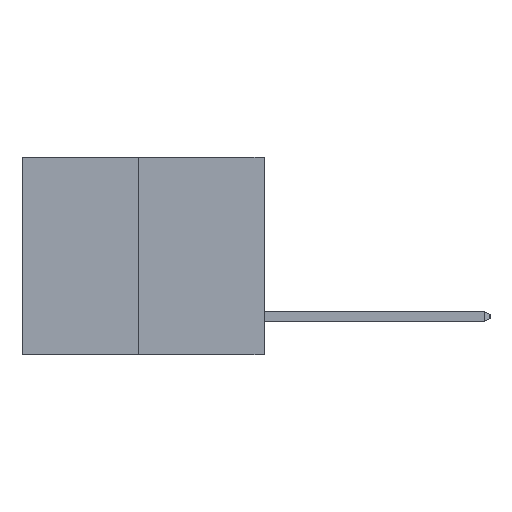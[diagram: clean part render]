
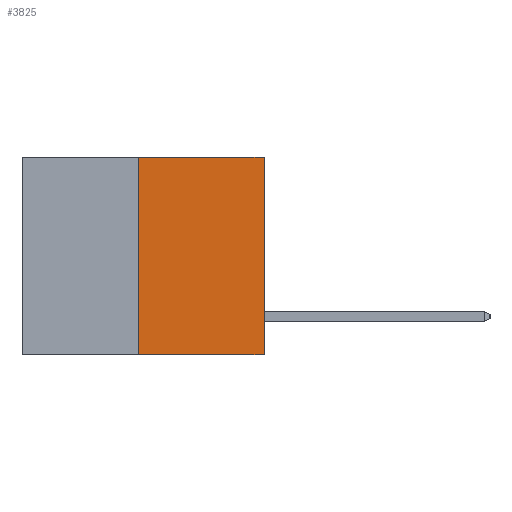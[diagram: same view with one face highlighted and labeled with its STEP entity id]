
A CAD part, left-side view. The second image highlights one B-rep face of the part: STEP entity #3825.
In plain terms, the highlighted planar face has unit normal (-1, 0, 0).
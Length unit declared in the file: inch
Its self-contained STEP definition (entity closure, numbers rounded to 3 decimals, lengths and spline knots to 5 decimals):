
#410 = ORIENTED_EDGE ( 'NONE', *, *, #24443, .F. ) ;
#1577 = CARTESIAN_POINT ( 'NONE',  ( 0., 0., 0. ) ) ;
#1878 = CARTESIAN_POINT ( 'NONE',  ( 0., 0.6, 0. ) ) ;
#3825 = ADVANCED_FACE ( 'NONE', ( #20770 ), #22673, .F. ) ;
#4087 = VECTOR ( 'NONE', #16035, 39.37008 ) ;
#5200 = VERTEX_POINT ( 'NONE', #17075 ) ;
#6329 = EDGE_LOOP ( 'NONE', ( #410, #20062, #16530, #17136 ) ) ;
#8845 = EDGE_CURVE ( 'NONE', #25019, #18686, #23222, .T. ) ;
#9444 = CARTESIAN_POINT ( 'NONE',  ( 0., 0.312, -0.49 ) ) ;
#9666 = CARTESIAN_POINT ( 'NONE',  ( 0., 0.6, -0.49 ) ) ;
#10748 = DIRECTION ( 'NONE',  ( 0., 0., 1. ) ) ;
#10788 = AXIS2_PLACEMENT_3D ( 'NONE', #15175, #15075, #24853 ) ;
#11562 = CARTESIAN_POINT ( 'NONE',  ( 0., 0.312, -0.49 ) ) ;
#12429 = VECTOR ( 'NONE', #10748, 39.37008 ) ;
#14781 = EDGE_CURVE ( 'NONE', #18686, #22151, #29075, .T. ) ;
#15075 = DIRECTION ( 'NONE',  ( 1., 0., 0. ) ) ;
#15175 = CARTESIAN_POINT ( 'NONE',  ( 0., 0.6, 0. ) ) ;
#15439 = LINE ( 'NONE', #1878, #19300 ) ;
#15719 = DIRECTION ( 'NONE',  ( 0., -1., 0. ) ) ;
#16035 = DIRECTION ( 'NONE',  ( 0., 0., 1. ) ) ;
#16257 = CARTESIAN_POINT ( 'NONE',  ( 0., 0., 0. ) ) ;
#16530 = ORIENTED_EDGE ( 'NONE', *, *, #14781, .T. ) ;
#17075 = CARTESIAN_POINT ( 'NONE',  ( 0., 0.312, 0. ) ) ;
#17136 = ORIENTED_EDGE ( 'NONE', *, *, #17328, .F. ) ;
#17212 = VECTOR ( 'NONE', #23010, 39.37008 ) ;
#17328 = EDGE_CURVE ( 'NONE', #5200, #22151, #15439, .T. ) ;
#18207 = LINE ( 'NONE', #11562, #4087 ) ;
#18686 = VERTEX_POINT ( 'NONE', #21791 ) ;
#19300 = VECTOR ( 'NONE', #15719, 39.37008 ) ;
#20062 = ORIENTED_EDGE ( 'NONE', *, *, #8845, .T. ) ;
#20770 = FACE_OUTER_BOUND ( 'NONE', #6329, .T. ) ;
#21791 = CARTESIAN_POINT ( 'NONE',  ( 0., 0., -0.49 ) ) ;
#22151 = VERTEX_POINT ( 'NONE', #16257 ) ;
#22673 = PLANE ( 'NONE',  #10788 ) ;
#23010 = DIRECTION ( 'NONE',  ( 0., -1., 0. ) ) ;
#23222 = LINE ( 'NONE', #9666, #17212 ) ;
#24443 = EDGE_CURVE ( 'NONE', #25019, #5200, #18207, .T. ) ;
#24853 = DIRECTION ( 'NONE',  ( 0., 0., -1. ) ) ;
#25019 = VERTEX_POINT ( 'NONE', #9444 ) ;
#29075 = LINE ( 'NONE', #1577, #12429 ) ;
